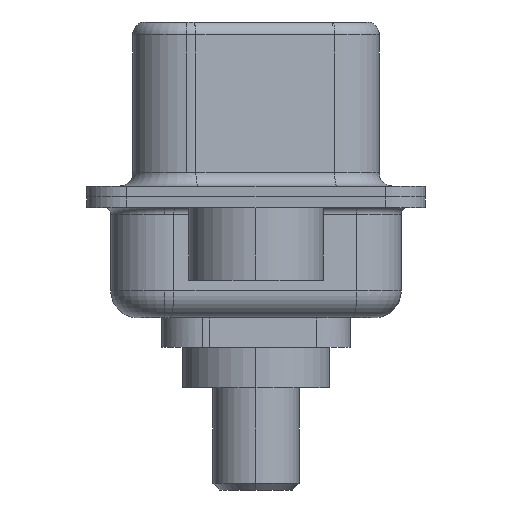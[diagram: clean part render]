
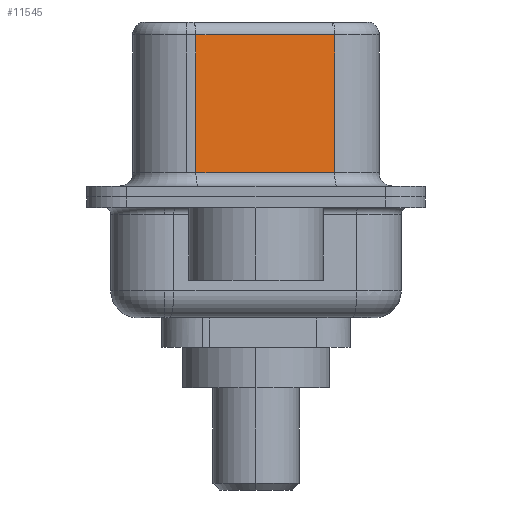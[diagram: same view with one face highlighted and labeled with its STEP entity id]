
A CAD part, left-side view. The second image highlights one B-rep face of the part: STEP entity #11545.
In plain terms, the highlighted planar face has unit normal (-0.985, -0.174, 0).
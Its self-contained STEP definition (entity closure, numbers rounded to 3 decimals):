
#580 = FACE_OUTER_BOUND ( 'NONE', #2379, .T. ) ;
#1264 = EDGE_CURVE ( 'NONE', #4434, #17929, #7620, .T. ) ;
#1471 = LINE ( 'NONE', #10197, #15557 ) ;
#1658 = LINE ( 'NONE', #4973, #2776 ) ;
#1714 = CARTESIAN_POINT ( 'NONE',  ( 4.58, -2.927, 0.9 ) ) ;
#2379 = EDGE_LOOP ( 'NONE', ( #9874, #7054, #18568, #12232 ) ) ;
#2776 = VECTOR ( 'NONE', #10917, 1000. ) ;
#3150 = DIRECTION ( 'NONE',  ( 0.174, -0.985, 0. ) ) ;
#3294 = CARTESIAN_POINT ( 'NONE',  ( 3.67, 2.233, 0.9 ) ) ;
#3418 = VERTEX_POINT ( 'NONE', #11500 ) ;
#3778 = EDGE_CURVE ( 'NONE', #16126, #4434, #1658, .T. ) ;
#4434 = VERTEX_POINT ( 'NONE', #3294 ) ;
#4973 = CARTESIAN_POINT ( 'NONE',  ( 3.67, 2.233, 6.52 ) ) ;
#4996 = EDGE_CURVE ( 'NONE', #3418, #17929, #1471, .T. ) ;
#6272 = DIRECTION ( 'NONE',  ( 0.985, 0.174, 0. ) ) ;
#6876 = CARTESIAN_POINT ( 'NONE',  ( 3.67, 2.233, 6.02 ) ) ;
#7054 = ORIENTED_EDGE ( 'NONE', *, *, #17361, .T. ) ;
#7620 = LINE ( 'NONE', #1714, #10131 ) ;
#7715 = CARTESIAN_POINT ( 'NONE',  ( 4.58, -2.927, 6.02 ) ) ;
#8015 = AXIS2_PLACEMENT_3D ( 'NONE', #14898, #6272, #10583 ) ;
#8695 = DIRECTION ( 'NONE',  ( 0., 0., -1. ) ) ;
#9181 = DIRECTION ( 'NONE',  ( -0.174, 0.985, 0. ) ) ;
#9489 = LINE ( 'NONE', #7715, #10153 ) ;
#9874 = ORIENTED_EDGE ( 'NONE', *, *, #4996, .F. ) ;
#10131 = VECTOR ( 'NONE', #3150, 1000. ) ;
#10153 = VECTOR ( 'NONE', #9181, 1000. ) ;
#10197 = CARTESIAN_POINT ( 'NONE',  ( 4.58, -2.927, 6.52 ) ) ;
#10583 = DIRECTION ( 'NONE',  ( -0.174, 0.985, 0. ) ) ;
#10653 = CARTESIAN_POINT ( 'NONE',  ( 4.58, -2.927, 0.9 ) ) ;
#10917 = DIRECTION ( 'NONE',  ( 0., 0., -1. ) ) ;
#11500 = CARTESIAN_POINT ( 'NONE',  ( 4.58, -2.927, 6.02 ) ) ;
#11545 = ADVANCED_FACE ( 'NONE', ( #580 ), #14963, .F. ) ;
#12232 = ORIENTED_EDGE ( 'NONE', *, *, #1264, .T. ) ;
#14898 = CARTESIAN_POINT ( 'NONE',  ( 4.58, -2.927, 6.52 ) ) ;
#14963 = PLANE ( 'NONE',  #8015 ) ;
#15557 = VECTOR ( 'NONE', #8695, 1000. ) ;
#16126 = VERTEX_POINT ( 'NONE', #6876 ) ;
#17361 = EDGE_CURVE ( 'NONE', #3418, #16126, #9489, .T. ) ;
#17929 = VERTEX_POINT ( 'NONE', #10653 ) ;
#18568 = ORIENTED_EDGE ( 'NONE', *, *, #3778, .T. ) ;
